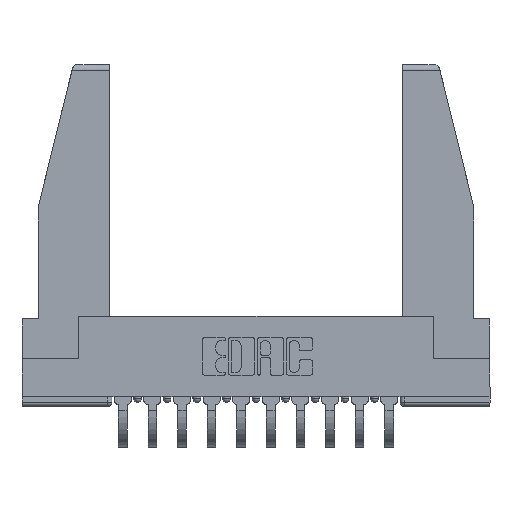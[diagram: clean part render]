
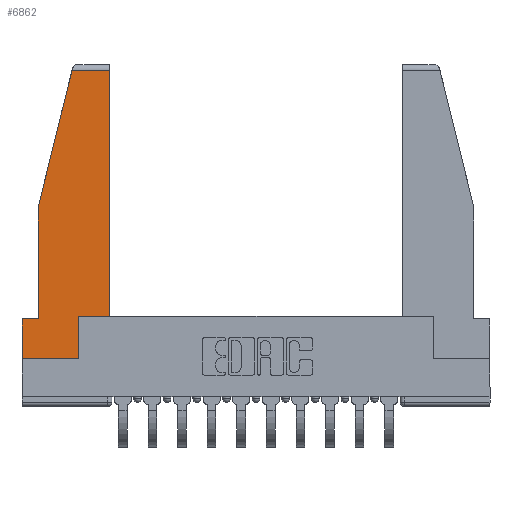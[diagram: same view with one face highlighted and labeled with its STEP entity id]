
A CAD part, top view. The second image highlights one B-rep face of the part: STEP entity #6862.
In plain terms, the highlighted planar face has unit normal (0, 0, 1).
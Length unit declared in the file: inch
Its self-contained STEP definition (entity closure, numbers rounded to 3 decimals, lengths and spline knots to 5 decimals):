
#995 = DIRECTION ( 'NONE',  ( -0.239, -0.971, 0. ) ) ;
#1117 = EDGE_CURVE ( 'NONE', #1908, #11580, #2316, .T. ) ;
#1155 = ORIENTED_EDGE ( 'NONE', *, *, #1117, .T. ) ;
#1165 = CARTESIAN_POINT ( 'NONE',  ( 0., 0., 0. ) ) ;
#1549 = EDGE_LOOP ( 'NONE', ( #1669, #8399, #3386, #11300, #3422, #16015, #3263, #1155, #3003 ) ) ;
#1669 = ORIENTED_EDGE ( 'NONE', *, *, #10767, .T. ) ;
#1736 = CARTESIAN_POINT ( 'NONE',  ( 0., 0.21, 0. ) ) ;
#1740 = CARTESIAN_POINT ( 'NONE',  ( 0.297, 0.223, 0. ) ) ;
#1908 = VERTEX_POINT ( 'NONE', #14035 ) ;
#2316 = LINE ( 'NONE', #14165, #14045 ) ;
#2392 = VERTEX_POINT ( 'NONE', #11690 ) ;
#2565 = DIRECTION ( 'NONE',  ( 0., 1., 0. ) ) ;
#2757 = DIRECTION ( 'NONE',  ( 0., -1., 0. ) ) ;
#2824 = VERTEX_POINT ( 'NONE', #7699 ) ;
#3003 = ORIENTED_EDGE ( 'NONE', *, *, #4095, .T. ) ;
#3190 = EDGE_CURVE ( 'NONE', #2824, #14032, #16606, .T. ) ;
#3263 = ORIENTED_EDGE ( 'NONE', *, *, #9871, .T. ) ;
#3386 = ORIENTED_EDGE ( 'NONE', *, *, #3190, .T. ) ;
#3422 = ORIENTED_EDGE ( 'NONE', *, *, #11073, .T. ) ;
#3473 = DIRECTION ( 'NONE',  ( 0., 1., 0. ) ) ;
#3558 = CARTESIAN_POINT ( 'NONE',  ( 0.271, 1.55, 0. ) ) ;
#4095 = EDGE_CURVE ( 'NONE', #11580, #12727, #16137, .T. ) ;
#4386 = EDGE_CURVE ( 'NONE', #14032, #14094, #4966, .T. ) ;
#4398 = DIRECTION ( 'NONE',  ( -1., 0., 0. ) ) ;
#4422 = CARTESIAN_POINT ( 'NONE',  ( 0.461, 1.52, 0. ) ) ;
#4524 = CARTESIAN_POINT ( 'NONE',  ( 0., 1.52, 0. ) ) ;
#4872 = DIRECTION ( 'NONE',  ( 0., -1., 0. ) ) ;
#4966 = LINE ( 'NONE', #7483, #8786 ) ;
#5163 = VECTOR ( 'NONE', #3473, 39.37008 ) ;
#5806 = CARTESIAN_POINT ( 'NONE',  ( 0.297, 0.223, 0. ) ) ;
#5893 = CARTESIAN_POINT ( 'NONE',  ( 0., 0., 0. ) ) ;
#6284 = CARTESIAN_POINT ( 'NONE',  ( 0.461, 0.223, 0. ) ) ;
#6862 = ADVANCED_FACE ( 'NONE', ( #8352 ), #10799, .T. ) ;
#7211 = VERTEX_POINT ( 'NONE', #1165 ) ;
#7483 = CARTESIAN_POINT ( 'NONE',  ( 0.086, 0.8, 0. ) ) ;
#7699 = CARTESIAN_POINT ( 'NONE',  ( 0.2636, 1.52, 0. ) ) ;
#8352 = FACE_OUTER_BOUND ( 'NONE', #1549, .T. ) ;
#8399 = ORIENTED_EDGE ( 'NONE', *, *, #14000, .T. ) ;
#8786 = VECTOR ( 'NONE', #4872, 39.37008 ) ;
#9380 = VECTOR ( 'NONE', #995, 39.37008 ) ;
#9453 = CARTESIAN_POINT ( 'NONE',  ( 0., 0., 0. ) ) ;
#9661 = LINE ( 'NONE', #4524, #14848 ) ;
#9699 = EDGE_CURVE ( 'NONE', #2392, #7211, #13385, .T. ) ;
#9721 = LINE ( 'NONE', #14903, #5163 ) ;
#9871 = EDGE_CURVE ( 'NONE', #7211, #1908, #12204, .T. ) ;
#10535 = VECTOR ( 'NONE', #4398, 39.37008 ) ;
#10715 = DIRECTION ( 'NONE',  ( 1., 0., 0. ) ) ;
#10731 = VERTEX_POINT ( 'NONE', #4422 ) ;
#10767 = EDGE_CURVE ( 'NONE', #12727, #10731, #9721, .T. ) ;
#10799 = PLANE ( 'NONE',  #12894 ) ;
#10878 = CARTESIAN_POINT ( 'NONE',  ( 0., 0.21, 0. ) ) ;
#10935 = DIRECTION ( 'NONE',  ( 1., 0., 0. ) ) ;
#11073 = EDGE_CURVE ( 'NONE', #14094, #2392, #15998, .T. ) ;
#11300 = ORIENTED_EDGE ( 'NONE', *, *, #4386, .T. ) ;
#11580 = VERTEX_POINT ( 'NONE', #1740 ) ;
#11690 = CARTESIAN_POINT ( 'NONE',  ( 0., 0.21, 0. ) ) ;
#11956 = VECTOR ( 'NONE', #15108, 39.37008 ) ;
#12204 = LINE ( 'NONE', #5893, #11956 ) ;
#12727 = VERTEX_POINT ( 'NONE', #6284 ) ;
#12894 = AXIS2_PLACEMENT_3D ( 'NONE', #9453, #15828, #10715 ) ;
#12897 = VECTOR ( 'NONE', #10935, 39.37008 ) ;
#13295 = VECTOR ( 'NONE', #2757, 39.37008 ) ;
#13385 = LINE ( 'NONE', #1736, #13295 ) ;
#14000 = EDGE_CURVE ( 'NONE', #10731, #2824, #9661, .T. ) ;
#14032 = VERTEX_POINT ( 'NONE', #16296 ) ;
#14035 = CARTESIAN_POINT ( 'NONE',  ( 0.297, 0., 0. ) ) ;
#14045 = VECTOR ( 'NONE', #2565, 39.37008 ) ;
#14094 = VERTEX_POINT ( 'NONE', #14159 ) ;
#14159 = CARTESIAN_POINT ( 'NONE',  ( 0.086, 0.21, 0. ) ) ;
#14165 = CARTESIAN_POINT ( 'NONE',  ( 0.297, 0., 0. ) ) ;
#14848 = VECTOR ( 'NONE', #16048, 39.37008 ) ;
#14903 = CARTESIAN_POINT ( 'NONE',  ( 0.461, 0.223, 0. ) ) ;
#15108 = DIRECTION ( 'NONE',  ( 1., 0., 0. ) ) ;
#15828 = DIRECTION ( 'NONE',  ( 0., 0., 1. ) ) ;
#15998 = LINE ( 'NONE', #10878, #10535 ) ;
#16015 = ORIENTED_EDGE ( 'NONE', *, *, #9699, .T. ) ;
#16048 = DIRECTION ( 'NONE',  ( -1., 0., 0. ) ) ;
#16137 = LINE ( 'NONE', #5806, #12897 ) ;
#16296 = CARTESIAN_POINT ( 'NONE',  ( 0.086, 0.8, 0. ) ) ;
#16606 = LINE ( 'NONE', #3558, #9380 ) ;
